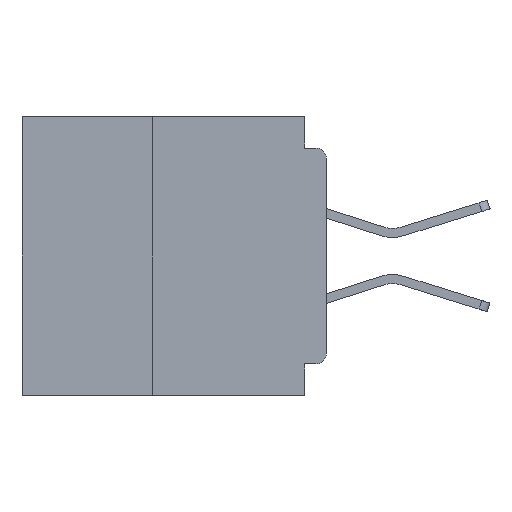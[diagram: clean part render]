
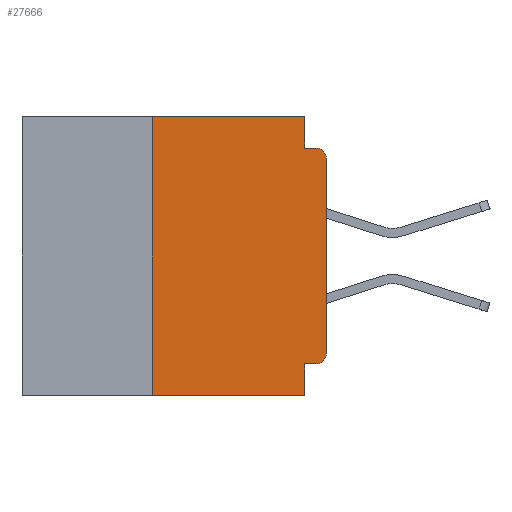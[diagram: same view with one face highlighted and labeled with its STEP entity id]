
A CAD part, left-side view. The second image highlights one B-rep face of the part: STEP entity #27666.
In plain terms, the highlighted planar face has unit normal (-1, 0, 0).
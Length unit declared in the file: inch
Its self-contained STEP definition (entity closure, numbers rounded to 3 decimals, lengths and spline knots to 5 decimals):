
#137 = EDGE_CURVE ( 'NONE', #16755, #28593, #7619, .T. ) ;
#675 = PLANE ( 'NONE',  #25521 ) ;
#1377 = CARTESIAN_POINT ( 'NONE',  ( 0., 0.031, -0.355 ) ) ;
#1736 = DIRECTION ( 'NONE',  ( 0., 0., -1. ) ) ;
#2380 = EDGE_CURVE ( 'NONE', #32964, #19485, #30659, .T. ) ;
#2835 = CARTESIAN_POINT ( 'NONE',  ( 0., 0., -0.045 ) ) ;
#3045 = CARTESIAN_POINT ( 'NONE',  ( 0., 0.25, -0.4 ) ) ;
#3072 = VERTEX_POINT ( 'NONE', #23141 ) ;
#3117 = CARTESIAN_POINT ( 'NONE',  ( 0., 0., -0.06 ) ) ;
#3558 = DIRECTION ( 'NONE',  ( 0., 0., -1. ) ) ;
#3815 = DIRECTION ( 'NONE',  ( 1., 0., 0. ) ) ;
#4057 = CARTESIAN_POINT ( 'NONE',  ( 0., 0.031, -0.4 ) ) ;
#4589 = CARTESIAN_POINT ( 'NONE',  ( 0., 0.015, -0.045 ) ) ;
#4641 = VECTOR ( 'NONE', #19467, 39.37008 ) ;
#5041 = EDGE_CURVE ( 'NONE', #37973, #20376, #23068, .T. ) ;
#5059 = EDGE_CURVE ( 'NONE', #16619, #28593, #22139, .T. ) ;
#5237 = CARTESIAN_POINT ( 'NONE',  ( 0., 0.031, -0.4 ) ) ;
#5997 = DIRECTION ( 'NONE',  ( 0., -1., 0. ) ) ;
#6009 = ORIENTED_EDGE ( 'NONE', *, *, #12996, .F. ) ;
#6156 = CARTESIAN_POINT ( 'NONE',  ( 0., 0.015, -0.06 ) ) ;
#6657 = VECTOR ( 'NONE', #1736, 39.37008 ) ;
#7275 = CARTESIAN_POINT ( 'NONE',  ( 0., 0.031, 0. ) ) ;
#7619 = LINE ( 'NONE', #4057, #6657 ) ;
#8633 = DIRECTION ( 'NONE',  ( 0., 1., 0. ) ) ;
#8765 = CARTESIAN_POINT ( 'NONE',  ( 0., 0., -0.355 ) ) ;
#9080 = ORIENTED_EDGE ( 'NONE', *, *, #5041, .F. ) ;
#9229 = DIRECTION ( 'NONE',  ( 0., 0., -1. ) ) ;
#9746 = ORIENTED_EDGE ( 'NONE', *, *, #2380, .T. ) ;
#9864 = CARTESIAN_POINT ( 'NONE',  ( 0., 0.437, 0. ) ) ;
#10041 = CARTESIAN_POINT ( 'NONE',  ( 0., 0.25, -0.4 ) ) ;
#10621 = EDGE_CURVE ( 'NONE', #29878, #30159, #20860, .T. ) ;
#10680 = LINE ( 'NONE', #8765, #24948 ) ;
#11054 = EDGE_CURVE ( 'NONE', #19485, #20376, #29799, .T. ) ;
#11250 = AXIS2_PLACEMENT_3D ( 'NONE', #6156, #27424, #9229 ) ;
#12634 = CARTESIAN_POINT ( 'NONE',  ( 0., 0.015, -0.34 ) ) ;
#12996 = EDGE_CURVE ( 'NONE', #3072, #16755, #10680, .T. ) ;
#14372 = FACE_OUTER_BOUND ( 'NONE', #21933, .T. ) ;
#14388 = EDGE_CURVE ( 'NONE', #30159, #37973, #38772, .T. ) ;
#14575 = VECTOR ( 'NONE', #34499, 39.37008 ) ;
#14830 = ORIENTED_EDGE ( 'NONE', *, *, #10621, .F. ) ;
#14996 = EDGE_CURVE ( 'NONE', #3072, #32964, #18063, .T. ) ;
#15166 = CARTESIAN_POINT ( 'NONE',  ( 0., 0.437, -0.4 ) ) ;
#15642 = DIRECTION ( 'NONE',  ( 0., 0., -1. ) ) ;
#15686 = CARTESIAN_POINT ( 'NONE',  ( 0., 0.031, 0. ) ) ;
#16389 = CARTESIAN_POINT ( 'NONE',  ( 0., 0.437, 0. ) ) ;
#16471 = CARTESIAN_POINT ( 'NONE',  ( 0., 0., -0.34 ) ) ;
#16619 = VERTEX_POINT ( 'NONE', #10041 ) ;
#16755 = VERTEX_POINT ( 'NONE', #1377 ) ;
#18063 = CIRCLE ( 'NONE', #28388, 0.015 ) ;
#19467 = DIRECTION ( 'NONE',  ( 0., -1., 0. ) ) ;
#19485 = VERTEX_POINT ( 'NONE', #3117 ) ;
#20376 = VERTEX_POINT ( 'NONE', #4589 ) ;
#20780 = ORIENTED_EDGE ( 'NONE', *, *, #11054, .T. ) ;
#20860 = LINE ( 'NONE', #16389, #4641 ) ;
#21175 = DIRECTION ( 'NONE',  ( 0., -1., 0. ) ) ;
#21933 = EDGE_LOOP ( 'NONE', ( #9746, #20780, #9080, #22940, #14830, #29014, #38606, #34411, #6009, #38882 ) ) ;
#22139 = LINE ( 'NONE', #15166, #24015 ) ;
#22940 = ORIENTED_EDGE ( 'NONE', *, *, #14388, .F. ) ;
#23068 = LINE ( 'NONE', #2835, #37987 ) ;
#23141 = CARTESIAN_POINT ( 'NONE',  ( 0., 0.015, -0.355 ) ) ;
#23530 = CARTESIAN_POINT ( 'NONE',  ( 0., 0.031, -0.045 ) ) ;
#23675 = LINE ( 'NONE', #3045, #31667 ) ;
#23884 = EDGE_CURVE ( 'NONE', #16619, #29878, #23675, .T. ) ;
#24015 = VECTOR ( 'NONE', #5997, 39.37008 ) ;
#24418 = DIRECTION ( 'NONE',  ( 0., 0., 1. ) ) ;
#24948 = VECTOR ( 'NONE', #8633, 39.37008 ) ;
#25150 = DIRECTION ( 'NONE',  ( 0., 0., -1. ) ) ;
#25521 = AXIS2_PLACEMENT_3D ( 'NONE', #9864, #3815, #25150 ) ;
#27424 = DIRECTION ( 'NONE',  ( -1., 0., 0. ) ) ;
#27666 = ADVANCED_FACE ( 'NONE', ( #14372 ), #675, .F. ) ;
#28388 = AXIS2_PLACEMENT_3D ( 'NONE', #12634, #33735, #15642 ) ;
#28593 = VERTEX_POINT ( 'NONE', #5237 ) ;
#29014 = ORIENTED_EDGE ( 'NONE', *, *, #23884, .F. ) ;
#29577 = CARTESIAN_POINT ( 'NONE',  ( 0., 0.25, 0. ) ) ;
#29799 = CIRCLE ( 'NONE', #11250, 0.015 ) ;
#29878 = VERTEX_POINT ( 'NONE', #29577 ) ;
#30159 = VERTEX_POINT ( 'NONE', #7275 ) ;
#30659 = LINE ( 'NONE', #33408, #14575 ) ;
#30924 = VECTOR ( 'NONE', #3558, 39.37008 ) ;
#31667 = VECTOR ( 'NONE', #24418, 39.37008 ) ;
#32964 = VERTEX_POINT ( 'NONE', #16471 ) ;
#33408 = CARTESIAN_POINT ( 'NONE',  ( 0., 0., 0. ) ) ;
#33735 = DIRECTION ( 'NONE',  ( -1., 0., 0. ) ) ;
#34411 = ORIENTED_EDGE ( 'NONE', *, *, #137, .F. ) ;
#34499 = DIRECTION ( 'NONE',  ( 0., 0., 1. ) ) ;
#37973 = VERTEX_POINT ( 'NONE', #23530 ) ;
#37987 = VECTOR ( 'NONE', #21175, 39.37008 ) ;
#38606 = ORIENTED_EDGE ( 'NONE', *, *, #5059, .T. ) ;
#38772 = LINE ( 'NONE', #15686, #30924 ) ;
#38882 = ORIENTED_EDGE ( 'NONE', *, *, #14996, .T. ) ;
